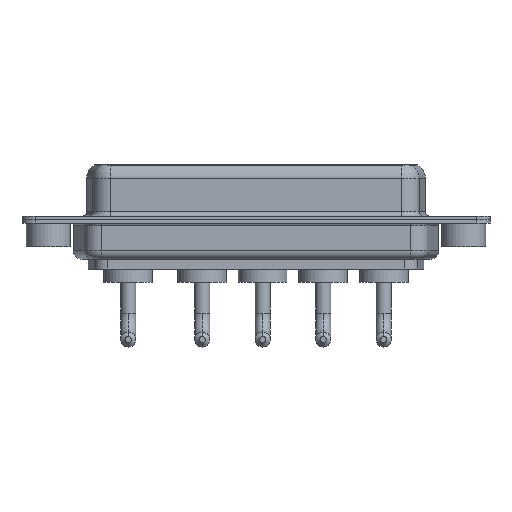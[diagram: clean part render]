
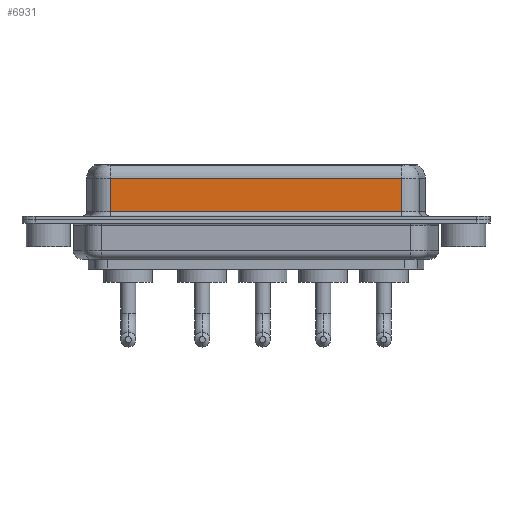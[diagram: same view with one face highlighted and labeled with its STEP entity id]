
A CAD part, front view. The second image highlights one B-rep face of the part: STEP entity #6931.
In plain terms, the highlighted planar face has unit normal (0, -1, 0).
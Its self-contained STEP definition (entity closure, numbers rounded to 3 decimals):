
#126 = CARTESIAN_POINT ( 'NONE',  ( 40.037, -3.95, 4.65 ) ) ;
#598 = PLANE ( 'NONE',  #6264 ) ;
#1348 = LINE ( 'NONE', #4309, #10663 ) ;
#2427 = CARTESIAN_POINT ( 'NONE',  ( 40.037, -3.95, 6.4 ) ) ;
#2456 = VECTOR ( 'NONE', #8580, 1000. ) ;
#3078 = EDGE_CURVE ( 'NONE', #4336, #3254, #1348, .T. ) ;
#3091 = VERTEX_POINT ( 'NONE', #8471 ) ;
#3254 = VERTEX_POINT ( 'NONE', #11550 ) ;
#3629 = LINE ( 'NONE', #5809, #10963 ) ;
#4308 = VERTEX_POINT ( 'NONE', #8986 ) ;
#4309 = CARTESIAN_POINT ( 'NONE',  ( 40.037, -3.95, 6.4 ) ) ;
#4336 = VERTEX_POINT ( 'NONE', #126 ) ;
#4348 = DIRECTION ( 'NONE',  ( 0., 1., 0. ) ) ;
#4598 = LINE ( 'NONE', #5824, #2456 ) ;
#5190 = EDGE_LOOP ( 'NONE', ( #12138, #12587, #5310, #12536 ) ) ;
#5310 = ORIENTED_EDGE ( 'NONE', *, *, #8358, .T. ) ;
#5809 = CARTESIAN_POINT ( 'NONE',  ( 40.037, -3.95, 0.9 ) ) ;
#5824 = CARTESIAN_POINT ( 'NONE',  ( 7.013, -3.95, 6.4 ) ) ;
#6264 = AXIS2_PLACEMENT_3D ( 'NONE', #2427, #4348, #11227 ) ;
#6298 = FACE_OUTER_BOUND ( 'NONE', #5190, .T. ) ;
#6727 = DIRECTION ( 'NONE',  ( 1., 0., 0. ) ) ;
#6931 = ADVANCED_FACE ( 'NONE', ( #6298 ), #598, .F. ) ;
#7466 = VECTOR ( 'NONE', #9172, 1000. ) ;
#8358 = EDGE_CURVE ( 'NONE', #3091, #4308, #4598, .T. ) ;
#8471 = CARTESIAN_POINT ( 'NONE',  ( 7.013, -3.95, 4.65 ) ) ;
#8580 = DIRECTION ( 'NONE',  ( 0., 0., -1. ) ) ;
#8986 = CARTESIAN_POINT ( 'NONE',  ( 7.013, -3.95, 0.9 ) ) ;
#9172 = DIRECTION ( 'NONE',  ( -1., 0., 0. ) ) ;
#9302 = DIRECTION ( 'NONE',  ( 0., 0., -1. ) ) ;
#10210 = EDGE_CURVE ( 'NONE', #4308, #3254, #3629, .T. ) ;
#10663 = VECTOR ( 'NONE', #9302, 1000. ) ;
#10963 = VECTOR ( 'NONE', #6727, 1000. ) ;
#11227 = DIRECTION ( 'NONE',  ( 0., 0., 1. ) ) ;
#11550 = CARTESIAN_POINT ( 'NONE',  ( 40.037, -3.95, 0.9 ) ) ;
#11764 = EDGE_CURVE ( 'NONE', #4336, #3091, #11880, .T. ) ;
#11880 = LINE ( 'NONE', #12009, #7466 ) ;
#12009 = CARTESIAN_POINT ( 'NONE',  ( 40.037, -3.95, 4.65 ) ) ;
#12138 = ORIENTED_EDGE ( 'NONE', *, *, #3078, .F. ) ;
#12536 = ORIENTED_EDGE ( 'NONE', *, *, #10210, .T. ) ;
#12587 = ORIENTED_EDGE ( 'NONE', *, *, #11764, .T. ) ;
